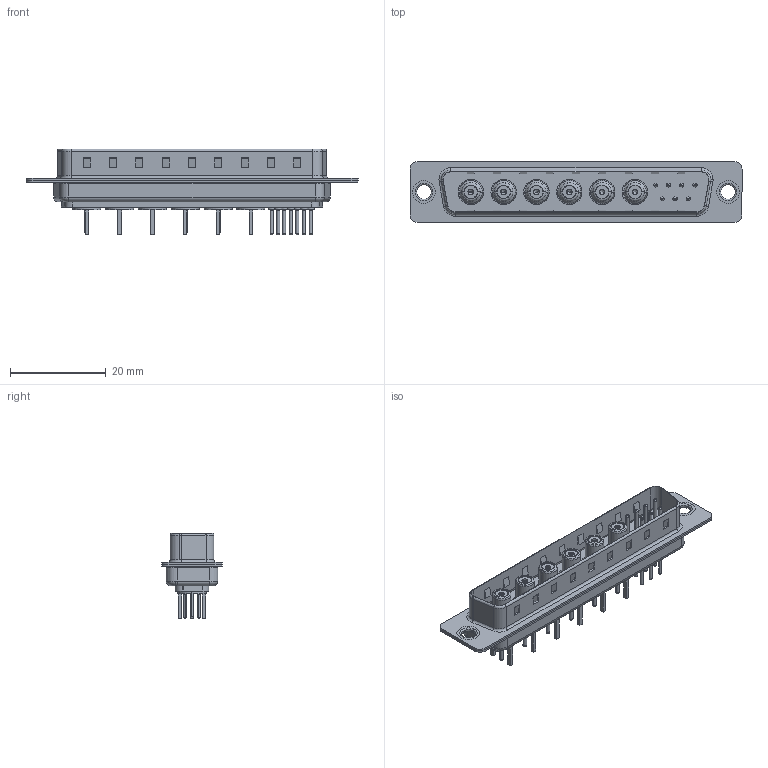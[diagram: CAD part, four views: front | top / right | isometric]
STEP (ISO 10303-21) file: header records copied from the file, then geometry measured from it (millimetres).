
FILE_DESCRIPTION (( 'STEP AP203' ), '1' );
FILE_NAME ('627-13W6224-5N1.STEP', '2019-05-28T19:58:37', ( '' ), ( '' ), 'SwSTEP 2.0', 'SolidWorks 2016', '' );
FILE_SCHEMA (( 'CONFIG_CONTROL_DESIGN' ));
Length unit declared in the file: millimetre
Products named in the file (13): 627Combo Contact Row 1_24; 627Combo Shell Front_37 Contacts; 627Combo Contact Row 2_24; 627Combo Thru Hole Rivet; 627-13W6224-5N1; Co-Ax Jack_Straight PC Tail; Insulator Socket; Insulator Socket 2; Locking Collar; Socket_Str; 627Combo Housing_13W6; Co-Ax Jack Assy_S; 627Combo Shell Rear_37 Contacts
Assembly tree (23 placements, depth 3):
  627-13W6224-5N1
    627Combo Housing_13W6
    627Combo Shell Rear_37 Contacts
    627Combo Shell Front_37 Contacts
    627Combo Thru Hole Rivet  x2
    Co-Ax Jack Assy_S  x6
      Co-Ax Jack_Straight PC Tail
      Insulator Socket
      Insulator Socket 2
      Locking Collar
      Socket_Str
    627Combo Contact Row 1_24  x4
    627Combo Contact Row 2_24  x3
Bounding box: 69.3 x 12.6 x 17.9 mm (x, y, z)
Volume: 3818.4 mm3; surface area: 11346 mm2
Topology: 42 solids, 42 shells, 1311 faces, 2987 edges, 1854 vertices
Faces by surface type: plane 534, cylinder 505, torus 194, cone 54, bspline 12, sphere 12
Entity records: 19906 total; most frequent: DIRECTION 3372, CARTESIAN_POINT 3197, ORIENTED_EDGE 2952, EDGE_CURVE 1476, AXIS2_PLACEMENT_3D 1282, VERTEX_POINT 930, VECTOR 808, LINE 808
